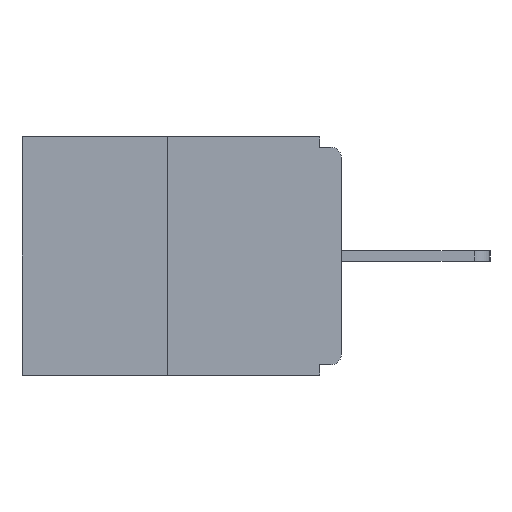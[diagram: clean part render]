
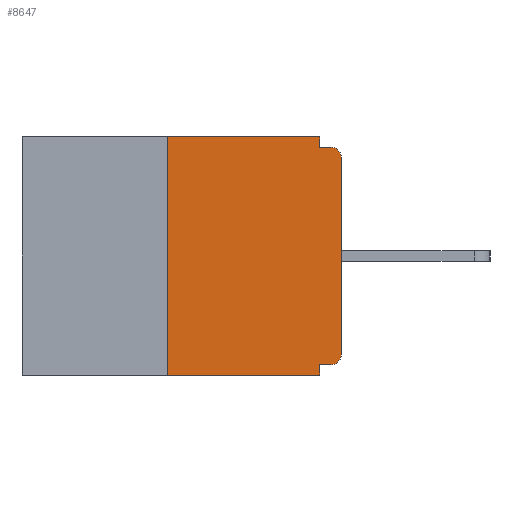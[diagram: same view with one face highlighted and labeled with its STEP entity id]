
A CAD part, left-side view. The second image highlights one B-rep face of the part: STEP entity #8647.
In plain terms, the highlighted planar face has unit normal (-1, 0, 0).
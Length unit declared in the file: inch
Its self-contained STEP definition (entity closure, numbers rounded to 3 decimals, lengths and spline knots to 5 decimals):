
#101 = DIRECTION ( 'NONE',  ( 0., 1., 0. ) ) ;
#279 = LINE ( 'NONE', #7395, #14056 ) ;
#355 = LINE ( 'NONE', #10886, #4828 ) ;
#549 = EDGE_CURVE ( 'NONE', #18795, #15166, #21345, .T. ) ;
#551 = ORIENTED_EDGE ( 'NONE', *, *, #9495, .T. ) ;
#599 = CARTESIAN_POINT ( 'NONE',  ( 0., 0.031, 0. ) ) ;
#667 = EDGE_CURVE ( 'NONE', #15166, #10750, #14018, .T. ) ;
#1061 = EDGE_CURVE ( 'NONE', #22313, #10750, #279, .T. ) ;
#1532 = EDGE_CURVE ( 'NONE', #18795, #7635, #20275, .T. ) ;
#1535 = VECTOR ( 'NONE', #7110, 39.37008 ) ;
#2358 = ORIENTED_EDGE ( 'NONE', *, *, #1061, .T. ) ;
#2713 = AXIS2_PLACEMENT_3D ( 'NONE', #3688, #5545, #10924 ) ;
#3610 = CARTESIAN_POINT ( 'NONE',  ( 0., 0.015, -0.015 ) ) ;
#3658 = CARTESIAN_POINT ( 'NONE',  ( 0., 0.015, -0.313 ) ) ;
#3688 = CARTESIAN_POINT ( 'NONE',  ( 0., 0.46, 0. ) ) ;
#4055 = VERTEX_POINT ( 'NONE', #3610 ) ;
#4082 = CARTESIAN_POINT ( 'NONE',  ( 0., 0., -0.03 ) ) ;
#4392 = CARTESIAN_POINT ( 'NONE',  ( 0., 0.031, -0.015 ) ) ;
#4489 = DIRECTION ( 'NONE',  ( 0., 0., -1. ) ) ;
#4547 = CARTESIAN_POINT ( 'NONE',  ( 0., 0.25, 0. ) ) ;
#4828 = VECTOR ( 'NONE', #18199, 39.37008 ) ;
#5038 = AXIS2_PLACEMENT_3D ( 'NONE', #18699, #18935, #4489 ) ;
#5446 = FACE_OUTER_BOUND ( 'NONE', #7864, .T. ) ;
#5490 = CARTESIAN_POINT ( 'NONE',  ( 0., 0., -0.328 ) ) ;
#5545 = DIRECTION ( 'NONE',  ( 1., 0., 0. ) ) ;
#6057 = VECTOR ( 'NONE', #101, 39.37008 ) ;
#6259 = EDGE_CURVE ( 'NONE', #11530, #4055, #18192, .T. ) ;
#7110 = DIRECTION ( 'NONE',  ( 0., 0., -1. ) ) ;
#7395 = CARTESIAN_POINT ( 'NONE',  ( 0., 0.46, -0.343 ) ) ;
#7635 = VERTEX_POINT ( 'NONE', #11691 ) ;
#7792 = DIRECTION ( 'NONE',  ( 0., 0., 1. ) ) ;
#7843 = LINE ( 'NONE', #13011, #18734 ) ;
#7864 = EDGE_LOOP ( 'NONE', ( #12435, #8806, #2358, #11701, #17864, #14947, #551, #13115, #10395, #22278 ) ) ;
#8051 = CARTESIAN_POINT ( 'NONE',  ( 0., 0.031, -0.328 ) ) ;
#8647 = ADVANCED_FACE ( 'NONE', ( #5446 ), #16588, .F. ) ;
#8683 = VERTEX_POINT ( 'NONE', #17796 ) ;
#8806 = ORIENTED_EDGE ( 'NONE', *, *, #17112, .F. ) ;
#9105 = VECTOR ( 'NONE', #21592, 39.37008 ) ;
#9117 = CARTESIAN_POINT ( 'NONE',  ( 0., 0., -0.015 ) ) ;
#9362 = EDGE_CURVE ( 'NONE', #8683, #19304, #355, .T. ) ;
#9495 = EDGE_CURVE ( 'NONE', #7635, #20585, #19214, .T. ) ;
#10395 = ORIENTED_EDGE ( 'NONE', *, *, #6259, .F. ) ;
#10750 = VERTEX_POINT ( 'NONE', #17989 ) ;
#10886 = CARTESIAN_POINT ( 'NONE',  ( 0., 0.46, 0. ) ) ;
#10924 = DIRECTION ( 'NONE',  ( 0., 0., -1. ) ) ;
#11530 = VERTEX_POINT ( 'NONE', #4392 ) ;
#11691 = CARTESIAN_POINT ( 'NONE',  ( 0., 0., -0.313 ) ) ;
#11701 = ORIENTED_EDGE ( 'NONE', *, *, #667, .F. ) ;
#12376 = CARTESIAN_POINT ( 'NONE',  ( 0., 0.25, -0.343 ) ) ;
#12435 = ORIENTED_EDGE ( 'NONE', *, *, #9362, .F. ) ;
#13011 = CARTESIAN_POINT ( 'NONE',  ( 0., 0.031, 0. ) ) ;
#13115 = ORIENTED_EDGE ( 'NONE', *, *, #18680, .T. ) ;
#13871 = CARTESIAN_POINT ( 'NONE',  ( 0., 0., 0. ) ) ;
#14018 = LINE ( 'NONE', #19589, #1535 ) ;
#14056 = VECTOR ( 'NONE', #21291, 39.37008 ) ;
#14345 = CIRCLE ( 'NONE', #5038, 0.015 ) ;
#14716 = EDGE_CURVE ( 'NONE', #19304, #11530, #7843, .T. ) ;
#14947 = ORIENTED_EDGE ( 'NONE', *, *, #1532, .T. ) ;
#15166 = VERTEX_POINT ( 'NONE', #8051 ) ;
#15628 = VECTOR ( 'NONE', #18981, 39.37008 ) ;
#16588 = PLANE ( 'NONE',  #2713 ) ;
#17112 = EDGE_CURVE ( 'NONE', #22313, #8683, #22263, .T. ) ;
#17539 = CARTESIAN_POINT ( 'NONE',  ( 0., 0.015, -0.328 ) ) ;
#17796 = CARTESIAN_POINT ( 'NONE',  ( 0., 0.25, 0. ) ) ;
#17864 = ORIENTED_EDGE ( 'NONE', *, *, #549, .F. ) ;
#17989 = CARTESIAN_POINT ( 'NONE',  ( 0., 0.031, -0.343 ) ) ;
#17990 = DIRECTION ( 'NONE',  ( -1., 0., 0. ) ) ;
#18102 = DIRECTION ( 'NONE',  ( 0., 0., -1. ) ) ;
#18192 = LINE ( 'NONE', #9117, #9105 ) ;
#18199 = DIRECTION ( 'NONE',  ( 0., -1., 0. ) ) ;
#18680 = EDGE_CURVE ( 'NONE', #20585, #4055, #14345, .T. ) ;
#18699 = CARTESIAN_POINT ( 'NONE',  ( 0., 0.015, -0.03 ) ) ;
#18734 = VECTOR ( 'NONE', #22318, 39.37008 ) ;
#18795 = VERTEX_POINT ( 'NONE', #17539 ) ;
#18935 = DIRECTION ( 'NONE',  ( -1., 0., 0. ) ) ;
#18981 = DIRECTION ( 'NONE',  ( 0., 0., 1. ) ) ;
#19214 = LINE ( 'NONE', #13871, #15628 ) ;
#19304 = VERTEX_POINT ( 'NONE', #599 ) ;
#19589 = CARTESIAN_POINT ( 'NONE',  ( 0., 0.031, -0.343 ) ) ;
#20275 = CIRCLE ( 'NONE', #22137, 0.015 ) ;
#20585 = VERTEX_POINT ( 'NONE', #4082 ) ;
#20676 = VECTOR ( 'NONE', #7792, 39.37008 ) ;
#21291 = DIRECTION ( 'NONE',  ( 0., -1., 0. ) ) ;
#21345 = LINE ( 'NONE', #5490, #6057 ) ;
#21592 = DIRECTION ( 'NONE',  ( 0., -1., 0. ) ) ;
#22137 = AXIS2_PLACEMENT_3D ( 'NONE', #3658, #17990, #18102 ) ;
#22263 = LINE ( 'NONE', #4547, #20676 ) ;
#22278 = ORIENTED_EDGE ( 'NONE', *, *, #14716, .F. ) ;
#22313 = VERTEX_POINT ( 'NONE', #12376 ) ;
#22318 = DIRECTION ( 'NONE',  ( 0., 0., -1. ) ) ;
